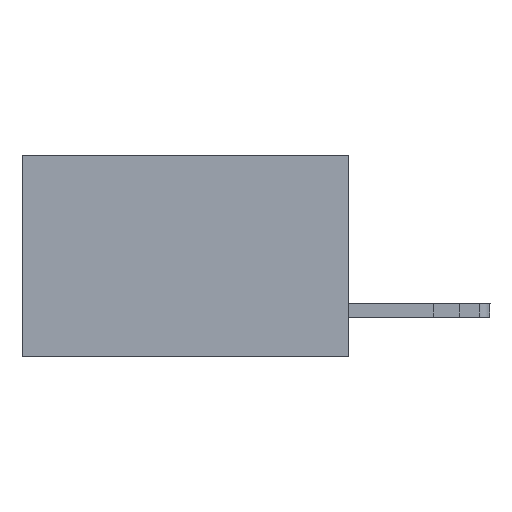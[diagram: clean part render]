
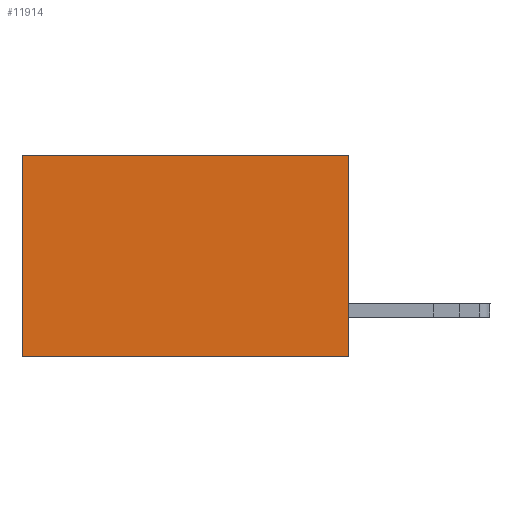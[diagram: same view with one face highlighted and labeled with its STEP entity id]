
A CAD part, left-side view. The second image highlights one B-rep face of the part: STEP entity #11914.
In plain terms, the highlighted planar face has unit normal (-1, 0, 0).
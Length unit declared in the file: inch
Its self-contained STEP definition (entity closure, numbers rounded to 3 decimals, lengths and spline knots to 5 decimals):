
#498 = CARTESIAN_POINT ( 'NONE',  ( 0.2615, 0., -0.37 ) ) ;
#2159 = ORIENTED_EDGE ( 'NONE', *, *, #18076, .F. ) ;
#2989 = VERTEX_POINT ( 'NONE', #4202 ) ;
#3231 = VERTEX_POINT ( 'NONE', #15715 ) ;
#3313 = LINE ( 'NONE', #6596, #19209 ) ;
#4202 = CARTESIAN_POINT ( 'NONE',  ( 0.2615, 0.6, -0.37 ) ) ;
#5002 = EDGE_CURVE ( 'NONE', #3231, #2989, #3313, .T. ) ;
#5144 = EDGE_LOOP ( 'NONE', ( #10179, #11266, #2159, #9882 ) ) ;
#5574 = VECTOR ( 'NONE', #17801, 39.37008 ) ;
#5721 = VERTEX_POINT ( 'NONE', #10515 ) ;
#6381 = CARTESIAN_POINT ( 'NONE',  ( 0.2615, 0., 0. ) ) ;
#6596 = CARTESIAN_POINT ( 'NONE',  ( 0.2615, 0., -0.37 ) ) ;
#7484 = DIRECTION ( 'NONE',  ( 0., 1., 0. ) ) ;
#7518 = LINE ( 'NONE', #498, #18503 ) ;
#7700 = PLANE ( 'NONE',  #15067 ) ;
#8229 = DIRECTION ( 'NONE',  ( 0., 0., -1. ) ) ;
#8987 = VERTEX_POINT ( 'NONE', #12914 ) ;
#9642 = EDGE_CURVE ( 'NONE', #5721, #8987, #19269, .T. ) ;
#9882 = ORIENTED_EDGE ( 'NONE', *, *, #9642, .T. ) ;
#10179 = ORIENTED_EDGE ( 'NONE', *, *, #18916, .T. ) ;
#10249 = FACE_OUTER_BOUND ( 'NONE', #5144, .T. ) ;
#10515 = CARTESIAN_POINT ( 'NONE',  ( 0.2615, 0., 0. ) ) ;
#10685 = DIRECTION ( 'NONE',  ( 0., 0., -1. ) ) ;
#10888 = VECTOR ( 'NONE', #12461, 39.37008 ) ;
#11126 = DIRECTION ( 'NONE',  ( 1., 0., 0. ) ) ;
#11266 = ORIENTED_EDGE ( 'NONE', *, *, #5002, .F. ) ;
#11914 = ADVANCED_FACE ( 'NONE', ( #10249 ), #7700, .F. ) ;
#12461 = DIRECTION ( 'NONE',  ( 0., 1., 0. ) ) ;
#12914 = CARTESIAN_POINT ( 'NONE',  ( 0.2615, 0.6, 0. ) ) ;
#15067 = AXIS2_PLACEMENT_3D ( 'NONE', #18191, #11126, #10685 ) ;
#15715 = CARTESIAN_POINT ( 'NONE',  ( 0.2615, 0., -0.37 ) ) ;
#16283 = CARTESIAN_POINT ( 'NONE',  ( 0.2615, 0.6, -0.37 ) ) ;
#17584 = LINE ( 'NONE', #16283, #5574 ) ;
#17801 = DIRECTION ( 'NONE',  ( 0., 0., -1. ) ) ;
#18076 = EDGE_CURVE ( 'NONE', #5721, #3231, #7518, .T. ) ;
#18191 = CARTESIAN_POINT ( 'NONE',  ( 0.2615, 0., -0.37 ) ) ;
#18503 = VECTOR ( 'NONE', #8229, 39.37008 ) ;
#18916 = EDGE_CURVE ( 'NONE', #8987, #2989, #17584, .T. ) ;
#19209 = VECTOR ( 'NONE', #7484, 39.37008 ) ;
#19269 = LINE ( 'NONE', #6381, #10888 ) ;
